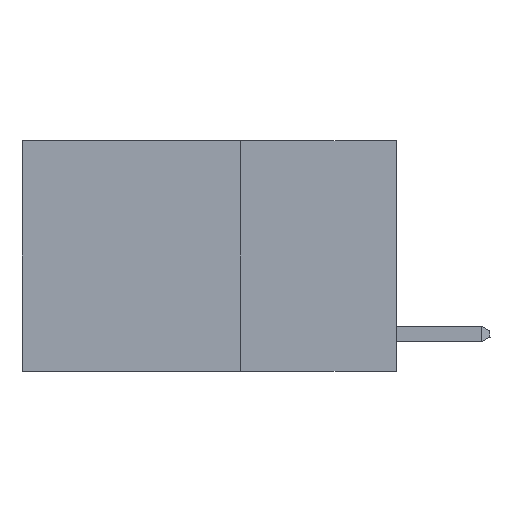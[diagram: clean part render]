
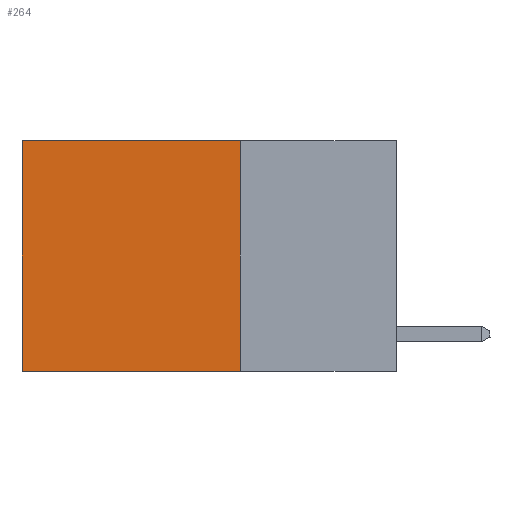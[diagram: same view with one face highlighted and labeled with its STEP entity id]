
A CAD part, left-side view. The second image highlights one B-rep face of the part: STEP entity #264.
In plain terms, the highlighted planar face has unit normal (-1, 0, 0).
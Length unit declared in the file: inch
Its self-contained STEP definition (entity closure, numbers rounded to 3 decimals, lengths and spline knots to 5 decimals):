
#264 = ADVANCED_FACE ( 'NONE', ( #22270 ), #1463, .F. ) ;
#273 = LINE ( 'NONE', #11527, #19915 ) ;
#480 = CARTESIAN_POINT ( 'NONE',  ( 0.2625, 0.6, 0. ) ) ;
#751 = DIRECTION ( 'NONE',  ( 0., 1., 0. ) ) ;
#1463 = PLANE ( 'NONE',  #11397 ) ;
#1670 = EDGE_CURVE ( 'NONE', #20223, #23264, #273, .T. ) ;
#2549 = CARTESIAN_POINT ( 'NONE',  ( 0.2625, 0.25, 0. ) ) ;
#3173 = ORIENTED_EDGE ( 'NONE', *, *, #1670, .F. ) ;
#3943 = DIRECTION ( 'NONE',  ( 0., 0., -1. ) ) ;
#5913 = DIRECTION ( 'NONE',  ( 0., 0., -1. ) ) ;
#5948 = EDGE_LOOP ( 'NONE', ( #10220, #7233, #3173, #8006 ) ) ;
#5977 = CARTESIAN_POINT ( 'NONE',  ( 0.2625, 0.25, -0.37 ) ) ;
#6370 = VECTOR ( 'NONE', #18957, 39.37008 ) ;
#6521 = VERTEX_POINT ( 'NONE', #14950 ) ;
#6952 = VECTOR ( 'NONE', #17045, 39.37008 ) ;
#7233 = ORIENTED_EDGE ( 'NONE', *, *, #15109, .F. ) ;
#8006 = ORIENTED_EDGE ( 'NONE', *, *, #14605, .T. ) ;
#8461 = CARTESIAN_POINT ( 'NONE',  ( 0.2625, 0.6, -0.37 ) ) ;
#10220 = ORIENTED_EDGE ( 'NONE', *, *, #15140, .T. ) ;
#11277 = LINE ( 'NONE', #480, #6370 ) ;
#11397 = AXIS2_PLACEMENT_3D ( 'NONE', #2549, #16951, #3943 ) ;
#11527 = CARTESIAN_POINT ( 'NONE',  ( 0.2625, 0.25, 0. ) ) ;
#11867 = LINE ( 'NONE', #5977, #6952 ) ;
#11948 = CARTESIAN_POINT ( 'NONE',  ( 0.2625, 0.25, 0. ) ) ;
#13021 = LINE ( 'NONE', #11948, #13603 ) ;
#13603 = VECTOR ( 'NONE', #751, 39.37008 ) ;
#14605 = EDGE_CURVE ( 'NONE', #20223, #6521, #13021, .T. ) ;
#14910 = CARTESIAN_POINT ( 'NONE',  ( 0.2625, 0.25, -0.37 ) ) ;
#14950 = CARTESIAN_POINT ( 'NONE',  ( 0.2625, 0.6, 0. ) ) ;
#15109 = EDGE_CURVE ( 'NONE', #23264, #22271, #11867, .T. ) ;
#15140 = EDGE_CURVE ( 'NONE', #6521, #22271, #11277, .T. ) ;
#16781 = CARTESIAN_POINT ( 'NONE',  ( 0.2625, 0.25, 0. ) ) ;
#16951 = DIRECTION ( 'NONE',  ( 1., 0., 0. ) ) ;
#17045 = DIRECTION ( 'NONE',  ( 0., 1., 0. ) ) ;
#18957 = DIRECTION ( 'NONE',  ( 0., 0., -1. ) ) ;
#19915 = VECTOR ( 'NONE', #5913, 39.37008 ) ;
#20223 = VERTEX_POINT ( 'NONE', #16781 ) ;
#22270 = FACE_OUTER_BOUND ( 'NONE', #5948, .T. ) ;
#22271 = VERTEX_POINT ( 'NONE', #8461 ) ;
#23264 = VERTEX_POINT ( 'NONE', #14910 ) ;
